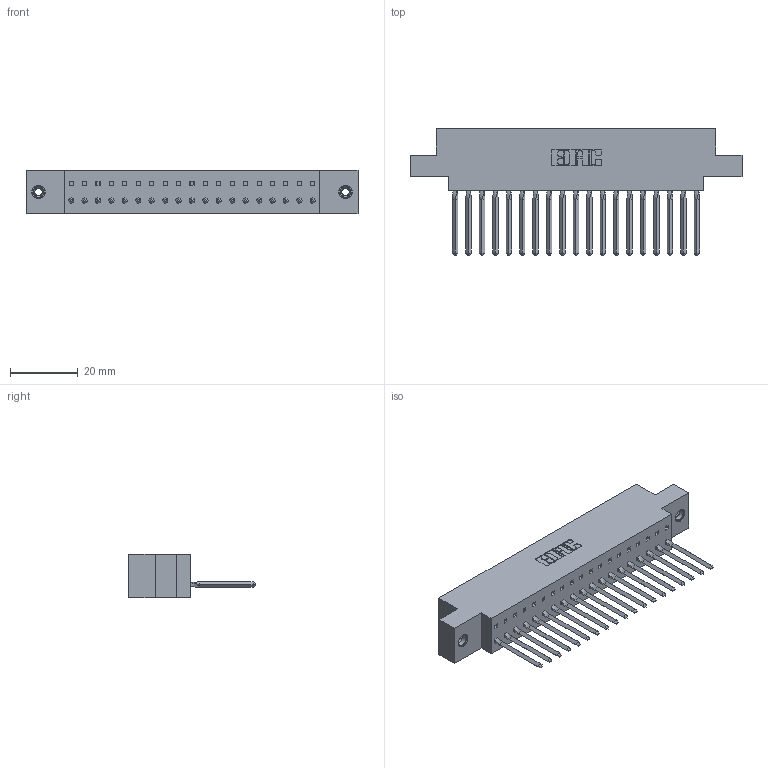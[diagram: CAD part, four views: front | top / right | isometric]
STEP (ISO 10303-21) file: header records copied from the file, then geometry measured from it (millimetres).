
FILE_DESCRIPTION (( 'STEP AP203' ), '1' );
FILE_NAME ('317-019-541-678.STEP', '2020-02-27T16:26:20', ( '' ), ( '' ), 'SwSTEP 2.0', 'SolidWorks 2016', '' );
FILE_SCHEMA (( 'CONFIG_CONTROL_DESIGN' ));
Length unit declared in the file: inch
Products named in the file (4): 317-290-002_541; 317 Part_.156 Dia - TI; 317-019-541-678; 345-250-001_345-250-003-102
Assembly tree (22 placements, depth 2):
  317-019-541-678
    317 Part_.156 Dia - TI
    317-290-002_541  x19
    345-250-001_345-250-003-102  x2
Bounding box: 97.99 x 37.34 x 12.7 mm (x, y, z)
Volume: 15177.5 mm3; surface area: 20701.5 mm2
Topology: 22 solids, 22 shells, 3050 faces, 8657 edges, 5624 vertices
Faces by surface type: plane 2446, cylinder 512, bspline 76, cone 12, torus 4
Entity records: 32799 total; most frequent: CARTESIAN_POINT 6429, ORIENTED_EDGE 5694, DIRECTION 4703, EDGE_CURVE 2847, VECTOR 2463, LINE 2463, VERTEX_POINT 1886, AXIS2_PLACEMENT_3D 1120
